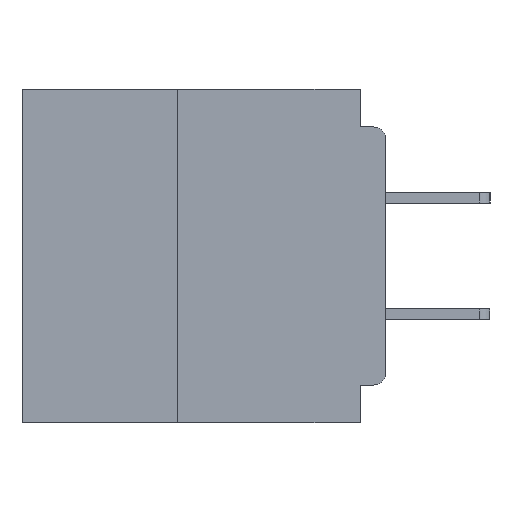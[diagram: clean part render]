
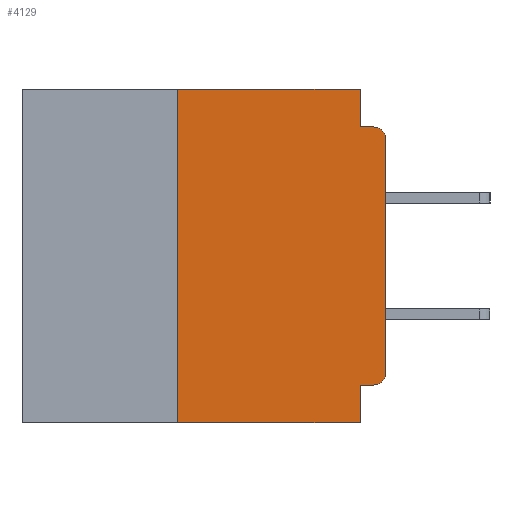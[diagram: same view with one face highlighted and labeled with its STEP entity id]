
A CAD part, left-side view. The second image highlights one B-rep face of the part: STEP entity #4129.
In plain terms, the highlighted planar face has unit normal (-1, 0, 0).
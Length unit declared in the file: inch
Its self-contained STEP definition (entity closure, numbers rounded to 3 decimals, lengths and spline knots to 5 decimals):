
#612 = VERTEX_POINT ( 'NONE', #16444 ) ;
#1608 = VECTOR ( 'NONE', #17354, 39.37008 ) ;
#1647 = VERTEX_POINT ( 'NONE', #17529 ) ;
#2582 = EDGE_CURVE ( 'NONE', #29668, #6112, #39340, .T. ) ;
#2769 = CARTESIAN_POINT ( 'NONE',  ( 0., 0.437, -0.4 ) ) ;
#3563 = EDGE_CURVE ( 'NONE', #9259, #20382, #8054, .T. ) ;
#4129 = ADVANCED_FACE ( 'NONE', ( #32197 ), #31676, .F. ) ;
#4557 = CARTESIAN_POINT ( 'NONE',  ( 0., 0.015, -0.06 ) ) ;
#5578 = CARTESIAN_POINT ( 'NONE',  ( 0., 0.015, -0.355 ) ) ;
#5657 = AXIS2_PLACEMENT_3D ( 'NONE', #31476, #31409, #31297 ) ;
#6112 = VERTEX_POINT ( 'NONE', #16267 ) ;
#6396 = VECTOR ( 'NONE', #10077, 39.37008 ) ;
#6408 = EDGE_CURVE ( 'NONE', #612, #1647, #26706, .T. ) ;
#6462 = DIRECTION ( 'NONE',  ( 0., -1., 0. ) ) ;
#6534 = DIRECTION ( 'NONE',  ( 0., -1., 0. ) ) ;
#6654 = VECTOR ( 'NONE', #48060, 39.37008 ) ;
#6664 = EDGE_CURVE ( 'NONE', #6112, #24764, #46025, .T. ) ;
#6972 = VERTEX_POINT ( 'NONE', #21451 ) ;
#8054 = LINE ( 'NONE', #27605, #1608 ) ;
#8345 = DIRECTION ( 'NONE',  ( 0., 0., -1. ) ) ;
#8431 = ORIENTED_EDGE ( 'NONE', *, *, #44835, .T. ) ;
#9259 = VERTEX_POINT ( 'NONE', #28039 ) ;
#9824 = DIRECTION ( 'NONE',  ( 0., 0., 1. ) ) ;
#10077 = DIRECTION ( 'NONE',  ( 0., 0., -1. ) ) ;
#10491 = CARTESIAN_POINT ( 'NONE',  ( 0., 0.437, 0. ) ) ;
#14008 = DIRECTION ( 'NONE',  ( 0., 1., 0. ) ) ;
#14172 = VERTEX_POINT ( 'NONE', #15441 ) ;
#14240 = VECTOR ( 'NONE', #6462, 39.37008 ) ;
#15375 = DIRECTION ( 'NONE',  ( -1., 0., 0. ) ) ;
#15441 = CARTESIAN_POINT ( 'NONE',  ( 0., 0.25, -0.4 ) ) ;
#16267 = CARTESIAN_POINT ( 'NONE',  ( 0., 0., -0.06 ) ) ;
#16444 = CARTESIAN_POINT ( 'NONE',  ( 0., 0.25, 0. ) ) ;
#16655 = ORIENTED_EDGE ( 'NONE', *, *, #47870, .F. ) ;
#17053 = ORIENTED_EDGE ( 'NONE', *, *, #3563, .F. ) ;
#17354 = DIRECTION ( 'NONE',  ( 0., 0., -1. ) ) ;
#17529 = CARTESIAN_POINT ( 'NONE',  ( 0., 0.031, 0. ) ) ;
#19840 = CARTESIAN_POINT ( 'NONE',  ( 0., 0.015, -0.045 ) ) ;
#20382 = VERTEX_POINT ( 'NONE', #33214 ) ;
#20950 = VECTOR ( 'NONE', #9824, 39.37008 ) ;
#21407 = VERTEX_POINT ( 'NONE', #5578 ) ;
#21451 = CARTESIAN_POINT ( 'NONE',  ( 0., 0.031, -0.045 ) ) ;
#21783 = EDGE_CURVE ( 'NONE', #21407, #29668, #41686, .T. ) ;
#24071 = LINE ( 'NONE', #32679, #6396 ) ;
#24764 = VERTEX_POINT ( 'NONE', #19840 ) ;
#25254 = EDGE_CURVE ( 'NONE', #6972, #24764, #41989, .T. ) ;
#25746 = LINE ( 'NONE', #2769, #35884 ) ;
#26185 = ORIENTED_EDGE ( 'NONE', *, *, #34865, .F. ) ;
#26706 = LINE ( 'NONE', #10491, #6654 ) ;
#27605 = CARTESIAN_POINT ( 'NONE',  ( 0., 0.031, -0.4 ) ) ;
#27660 = ORIENTED_EDGE ( 'NONE', *, *, #6408, .F. ) ;
#28008 = CARTESIAN_POINT ( 'NONE',  ( 0., 0., -0.34 ) ) ;
#28039 = CARTESIAN_POINT ( 'NONE',  ( 0., 0.031, -0.355 ) ) ;
#28104 = CARTESIAN_POINT ( 'NONE',  ( 0., 0., 0. ) ) ;
#28567 = EDGE_LOOP ( 'NONE', ( #38668, #32099, #31660, #31300, #27660, #26185, #8431, #17053, #16655, #29207 ) ) ;
#29180 = DIRECTION ( 'NONE',  ( 0., 0., 1. ) ) ;
#29207 = ORIENTED_EDGE ( 'NONE', *, *, #21783, .T. ) ;
#29668 = VERTEX_POINT ( 'NONE', #28008 ) ;
#30905 = DIRECTION ( 'NONE',  ( -1., 0., 0. ) ) ;
#31014 = LINE ( 'NONE', #39828, #20950 ) ;
#31297 = DIRECTION ( 'NONE',  ( 0., 0., -1. ) ) ;
#31300 = ORIENTED_EDGE ( 'NONE', *, *, #39874, .F. ) ;
#31409 = DIRECTION ( 'NONE',  ( 1., 0., 0. ) ) ;
#31476 = CARTESIAN_POINT ( 'NONE',  ( 0., 0.437, 0. ) ) ;
#31660 = ORIENTED_EDGE ( 'NONE', *, *, #25254, .F. ) ;
#31676 = PLANE ( 'NONE',  #5657 ) ;
#32099 = ORIENTED_EDGE ( 'NONE', *, *, #6664, .T. ) ;
#32197 = FACE_OUTER_BOUND ( 'NONE', #28567, .T. ) ;
#32679 = CARTESIAN_POINT ( 'NONE',  ( 0., 0.031, 0. ) ) ;
#32852 = CARTESIAN_POINT ( 'NONE',  ( 0., 0., -0.045 ) ) ;
#33214 = CARTESIAN_POINT ( 'NONE',  ( 0., 0.031, -0.4 ) ) ;
#34423 = VECTOR ( 'NONE', #14008, 39.37008 ) ;
#34865 = EDGE_CURVE ( 'NONE', #14172, #612, #31014, .T. ) ;
#35884 = VECTOR ( 'NONE', #6534, 39.37008 ) ;
#36098 = AXIS2_PLACEMENT_3D ( 'NONE', #4557, #30905, #8345 ) ;
#38031 = CARTESIAN_POINT ( 'NONE',  ( 0., 0.015, -0.34 ) ) ;
#38668 = ORIENTED_EDGE ( 'NONE', *, *, #2582, .T. ) ;
#39340 = LINE ( 'NONE', #28104, #46853 ) ;
#39828 = CARTESIAN_POINT ( 'NONE',  ( 0., 0.25, -0.4 ) ) ;
#39874 = EDGE_CURVE ( 'NONE', #1647, #6972, #24071, .T. ) ;
#40406 = CARTESIAN_POINT ( 'NONE',  ( 0., 0., -0.355 ) ) ;
#41686 = CIRCLE ( 'NONE', #45068, 0.015 ) ;
#41767 = DIRECTION ( 'NONE',  ( 0., 0., -1. ) ) ;
#41989 = LINE ( 'NONE', #32852, #14240 ) ;
#44835 = EDGE_CURVE ( 'NONE', #14172, #20382, #25746, .T. ) ;
#45068 = AXIS2_PLACEMENT_3D ( 'NONE', #38031, #15375, #41767 ) ;
#45489 = LINE ( 'NONE', #40406, #34423 ) ;
#46025 = CIRCLE ( 'NONE', #36098, 0.015 ) ;
#46853 = VECTOR ( 'NONE', #29180, 39.37008 ) ;
#47870 = EDGE_CURVE ( 'NONE', #21407, #9259, #45489, .T. ) ;
#48060 = DIRECTION ( 'NONE',  ( 0., -1., 0. ) ) ;
